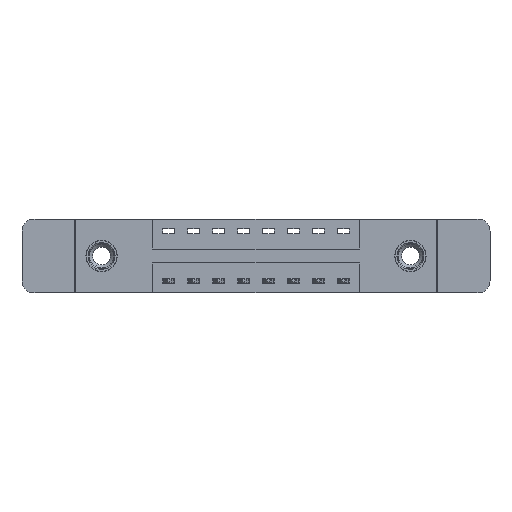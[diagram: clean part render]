
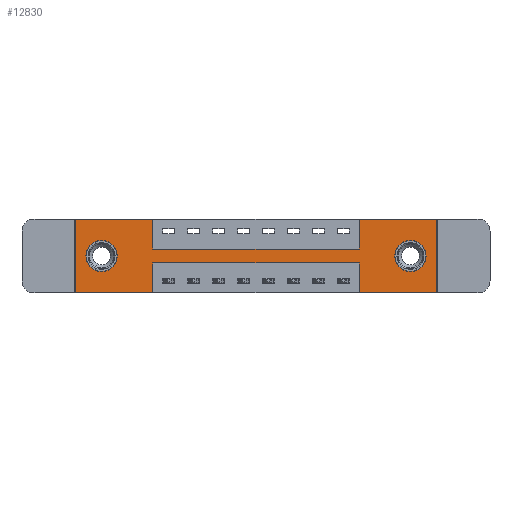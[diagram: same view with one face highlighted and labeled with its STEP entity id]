
A CAD part, front view. The second image highlights one B-rep face of the part: STEP entity #12830.
In plain terms, the highlighted planar face has unit normal (0, -1, 0).
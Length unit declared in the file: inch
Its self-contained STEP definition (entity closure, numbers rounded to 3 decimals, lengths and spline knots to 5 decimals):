
#36 = DIRECTION ( 'NONE',  ( 0., 1., 0. ) ) ;
#212 = CIRCLE ( 'NONE', #13801, 0.078 ) ;
#402 = DIRECTION ( 'NONE',  ( 1., 0., 0. ) ) ;
#416 = CARTESIAN_POINT ( 'NONE',  ( 0.3875, 0., -0.15 ) ) ;
#623 = ORIENTED_EDGE ( 'NONE', *, *, #10149, .F. ) ;
#809 = FACE_BOUND ( 'NONE', #6856, .T. ) ;
#820 = CARTESIAN_POINT ( 'NONE',  ( 0.1325, 0., -0.185 ) ) ;
#1088 = DIRECTION ( 'NONE',  ( 0., 0., 1. ) ) ;
#1117 = EDGE_CURVE ( 'NONE', #11633, #14490, #10348, .T. ) ;
#1225 = VECTOR ( 'NONE', #1500, 39.37008 ) ;
#1273 = LINE ( 'NONE', #416, #11716 ) ;
#1350 = CARTESIAN_POINT ( 'NONE',  ( 0.3875, 0., 0. ) ) ;
#1500 = DIRECTION ( 'NONE',  ( 0., 0., -1. ) ) ;
#1550 = CARTESIAN_POINT ( 'NONE',  ( 0.3875, 0., -0.37 ) ) ;
#1603 = CIRCLE ( 'NONE', #5068, 0.078 ) ;
#1736 = CARTESIAN_POINT ( 'NONE',  ( 0.3875, 0., -0.22 ) ) ;
#1751 = EDGE_CURVE ( 'NONE', #13718, #8251, #14001, .T. ) ;
#1825 = VERTEX_POINT ( 'NONE', #5698 ) ;
#2027 = PLANE ( 'NONE',  #11070 ) ;
#2082 = CARTESIAN_POINT ( 'NONE',  ( 1.4225, 0., 0. ) ) ;
#2383 = VERTEX_POINT ( 'NONE', #8867 ) ;
#2398 = LINE ( 'NONE', #13567, #10738 ) ;
#2424 = ORIENTED_EDGE ( 'NONE', *, *, #5687, .T. ) ;
#2638 = ORIENTED_EDGE ( 'NONE', *, *, #8152, .F. ) ;
#2885 = CARTESIAN_POINT ( 'NONE',  ( 0.3875, 0., -0.15 ) ) ;
#2969 = LINE ( 'NONE', #1550, #1225 ) ;
#3105 = FACE_OUTER_BOUND ( 'NONE', #12784, .T. ) ;
#3191 = DIRECTION ( 'NONE',  ( 0., 0., 1. ) ) ;
#3205 = EDGE_CURVE ( 'NONE', #1825, #13912, #11986, .T. ) ;
#3292 = VECTOR ( 'NONE', #14060, 39.37008 ) ;
#3353 = VECTOR ( 'NONE', #12870, 39.37008 ) ;
#3373 = ORIENTED_EDGE ( 'NONE', *, *, #6525, .F. ) ;
#3433 = ORIENTED_EDGE ( 'NONE', *, *, #12984, .F. ) ;
#3518 = CARTESIAN_POINT ( 'NONE',  ( 0.1325, 0., -0.185 ) ) ;
#3724 = VERTEX_POINT ( 'NONE', #14093 ) ;
#3831 = DIRECTION ( 'NONE',  ( 0., 0., -1. ) ) ;
#3896 = AXIS2_PLACEMENT_3D ( 'NONE', #820, #8780, #9913 ) ;
#3911 = ORIENTED_EDGE ( 'NONE', *, *, #9863, .T. ) ;
#4018 = VERTEX_POINT ( 'NONE', #14482 ) ;
#4062 = CARTESIAN_POINT ( 'NONE',  ( 0.1325, 0., -0.263 ) ) ;
#4114 = ORIENTED_EDGE ( 'NONE', *, *, #11052, .F. ) ;
#4125 = DIRECTION ( 'NONE',  ( 0., -1., 0. ) ) ;
#4727 = ORIENTED_EDGE ( 'NONE', *, *, #8470, .F. ) ;
#4832 = CARTESIAN_POINT ( 'NONE',  ( 1.6775, 0., -0.263 ) ) ;
#4989 = CARTESIAN_POINT ( 'NONE',  ( 0., 0., -0.37 ) ) ;
#5068 = AXIS2_PLACEMENT_3D ( 'NONE', #7082, #8238, #11522 ) ;
#5177 = DIRECTION ( 'NONE',  ( 0., 0., -1. ) ) ;
#5196 = VERTEX_POINT ( 'NONE', #4062 ) ;
#5451 = CARTESIAN_POINT ( 'NONE',  ( 1.4225, 0., -0.22 ) ) ;
#5456 = CARTESIAN_POINT ( 'NONE',  ( 0., 0., -0.37 ) ) ;
#5517 = CARTESIAN_POINT ( 'NONE',  ( 0.1325, 0., -0.107 ) ) ;
#5687 = EDGE_CURVE ( 'NONE', #9586, #5196, #13005, .T. ) ;
#5698 = CARTESIAN_POINT ( 'NONE',  ( 1.4225, 0., -0.37 ) ) ;
#5809 = VERTEX_POINT ( 'NONE', #8716 ) ;
#5927 = EDGE_CURVE ( 'NONE', #13779, #5809, #212, .T. ) ;
#6172 = CIRCLE ( 'NONE', #6371, 0.078 ) ;
#6371 = AXIS2_PLACEMENT_3D ( 'NONE', #3518, #14421, #3191 ) ;
#6525 = EDGE_CURVE ( 'NONE', #9449, #4018, #1273, .T. ) ;
#6708 = VERTEX_POINT ( 'NONE', #14434 ) ;
#6820 = ORIENTED_EDGE ( 'NONE', *, *, #5927, .T. ) ;
#6856 = EDGE_LOOP ( 'NONE', ( #2424, #12807 ) ) ;
#6903 = CARTESIAN_POINT ( 'NONE',  ( 1.6775, 0., -0.185 ) ) ;
#6912 = ORIENTED_EDGE ( 'NONE', *, *, #9147, .F. ) ;
#6962 = VECTOR ( 'NONE', #402, 39.37008 ) ;
#7082 = CARTESIAN_POINT ( 'NONE',  ( 1.6775, 0., -0.185 ) ) ;
#7390 = CARTESIAN_POINT ( 'NONE',  ( 1.4225, 0., -0.37 ) ) ;
#7600 = VECTOR ( 'NONE', #5177, 39.37008 ) ;
#7775 = VECTOR ( 'NONE', #14166, 39.37008 ) ;
#8144 = EDGE_CURVE ( 'NONE', #5196, #9586, #6172, .T. ) ;
#8152 = EDGE_CURVE ( 'NONE', #2383, #1825, #14020, .T. ) ;
#8238 = DIRECTION ( 'NONE',  ( 0., 1., 0. ) ) ;
#8251 = VERTEX_POINT ( 'NONE', #1350 ) ;
#8388 = DIRECTION ( 'NONE',  ( 1., 0., 0. ) ) ;
#8470 = EDGE_CURVE ( 'NONE', #14490, #2383, #14543, .T. ) ;
#8521 = CARTESIAN_POINT ( 'NONE',  ( 0.3875, 0., 0. ) ) ;
#8640 = VECTOR ( 'NONE', #9060, 39.37008 ) ;
#8716 = CARTESIAN_POINT ( 'NONE',  ( 1.6775, 0., -0.107 ) ) ;
#8780 = DIRECTION ( 'NONE',  ( 0., 1., 0. ) ) ;
#8867 = CARTESIAN_POINT ( 'NONE',  ( 1.81, 0., -0.37 ) ) ;
#8949 = ORIENTED_EDGE ( 'NONE', *, *, #1117, .F. ) ;
#8993 = DIRECTION ( 'NONE',  ( 1., 0., 0. ) ) ;
#9060 = DIRECTION ( 'NONE',  ( 0., 0., 1. ) ) ;
#9147 = EDGE_CURVE ( 'NONE', #13912, #11094, #10335, .T. ) ;
#9319 = ORIENTED_EDGE ( 'NONE', *, *, #1751, .F. ) ;
#9448 = VECTOR ( 'NONE', #10602, 39.37008 ) ;
#9449 = VERTEX_POINT ( 'NONE', #2885 ) ;
#9493 = CARTESIAN_POINT ( 'NONE',  ( 1.4225, 0., 0. ) ) ;
#9552 = EDGE_LOOP ( 'NONE', ( #3911, #6820 ) ) ;
#9586 = VERTEX_POINT ( 'NONE', #5517 ) ;
#9645 = ORIENTED_EDGE ( 'NONE', *, *, #12959, .F. ) ;
#9863 = EDGE_CURVE ( 'NONE', #5809, #13779, #1603, .T. ) ;
#9913 = DIRECTION ( 'NONE',  ( 0., 0., 1. ) ) ;
#9949 = CARTESIAN_POINT ( 'NONE',  ( 1.81, 0., 0. ) ) ;
#10052 = FACE_BOUND ( 'NONE', #9552, .T. ) ;
#10096 = LINE ( 'NONE', #13111, #7775 ) ;
#10149 = EDGE_CURVE ( 'NONE', #8251, #9449, #10304, .T. ) ;
#10304 = LINE ( 'NONE', #8521, #12419 ) ;
#10335 = LINE ( 'NONE', #10391, #9448 ) ;
#10348 = LINE ( 'NONE', #12911, #6962 ) ;
#10391 = CARTESIAN_POINT ( 'NONE',  ( 0.3875, 0., -0.22 ) ) ;
#10602 = DIRECTION ( 'NONE',  ( -1., 0., 0. ) ) ;
#10709 = EDGE_CURVE ( 'NONE', #11094, #3724, #2969, .T. ) ;
#10738 = VECTOR ( 'NONE', #1088, 39.37008 ) ;
#11052 = EDGE_CURVE ( 'NONE', #3724, #6708, #10096, .T. ) ;
#11070 = AXIS2_PLACEMENT_3D ( 'NONE', #5456, #4125, #14502 ) ;
#11094 = VERTEX_POINT ( 'NONE', #1736 ) ;
#11170 = ORIENTED_EDGE ( 'NONE', *, *, #3205, .F. ) ;
#11398 = DIRECTION ( 'NONE',  ( 0., 0., -1. ) ) ;
#11522 = DIRECTION ( 'NONE',  ( 0., 0., -1. ) ) ;
#11633 = VERTEX_POINT ( 'NONE', #9493 ) ;
#11716 = VECTOR ( 'NONE', #8388, 39.37008 ) ;
#11984 = CARTESIAN_POINT ( 'NONE',  ( 1.81, 0., 0. ) ) ;
#11986 = LINE ( 'NONE', #7390, #3292 ) ;
#12419 = VECTOR ( 'NONE', #3831, 39.37008 ) ;
#12507 = LINE ( 'NONE', #2082, #8640 ) ;
#12784 = EDGE_LOOP ( 'NONE', ( #13587, #6912, #11170, #2638, #4727, #8949, #3433, #3373, #623, #9319, #9645, #4114 ) ) ;
#12807 = ORIENTED_EDGE ( 'NONE', *, *, #8144, .T. ) ;
#12830 = ADVANCED_FACE ( 'NONE', ( #10052, #809, #3105 ), #2027, .T. ) ;
#12870 = DIRECTION ( 'NONE',  ( -1., 0., 0. ) ) ;
#12911 = CARTESIAN_POINT ( 'NONE',  ( 0., 0., 0. ) ) ;
#12959 = EDGE_CURVE ( 'NONE', #6708, #13718, #2398, .T. ) ;
#12984 = EDGE_CURVE ( 'NONE', #4018, #11633, #12507, .T. ) ;
#13005 = CIRCLE ( 'NONE', #3896, 0.078 ) ;
#13111 = CARTESIAN_POINT ( 'NONE',  ( 0., 0., -0.37 ) ) ;
#13439 = CARTESIAN_POINT ( 'NONE',  ( 0., 0., 0. ) ) ;
#13567 = CARTESIAN_POINT ( 'NONE',  ( 0., 0., 0. ) ) ;
#13587 = ORIENTED_EDGE ( 'NONE', *, *, #10709, .F. ) ;
#13718 = VERTEX_POINT ( 'NONE', #14065 ) ;
#13779 = VERTEX_POINT ( 'NONE', #4832 ) ;
#13801 = AXIS2_PLACEMENT_3D ( 'NONE', #6903, #36, #11398 ) ;
#13912 = VERTEX_POINT ( 'NONE', #5451 ) ;
#14001 = LINE ( 'NONE', #13439, #14528 ) ;
#14020 = LINE ( 'NONE', #4989, #3353 ) ;
#14060 = DIRECTION ( 'NONE',  ( 0., 0., 1. ) ) ;
#14065 = CARTESIAN_POINT ( 'NONE',  ( 0., 0., 0. ) ) ;
#14093 = CARTESIAN_POINT ( 'NONE',  ( 0.3875, 0., -0.37 ) ) ;
#14166 = DIRECTION ( 'NONE',  ( -1., 0., 0. ) ) ;
#14421 = DIRECTION ( 'NONE',  ( 0., 1., 0. ) ) ;
#14434 = CARTESIAN_POINT ( 'NONE',  ( 0., 0., -0.37 ) ) ;
#14482 = CARTESIAN_POINT ( 'NONE',  ( 1.4225, 0., -0.15 ) ) ;
#14490 = VERTEX_POINT ( 'NONE', #11984 ) ;
#14502 = DIRECTION ( 'NONE',  ( 0., 0., -1. ) ) ;
#14528 = VECTOR ( 'NONE', #8993, 39.37008 ) ;
#14543 = LINE ( 'NONE', #9949, #7600 ) ;
